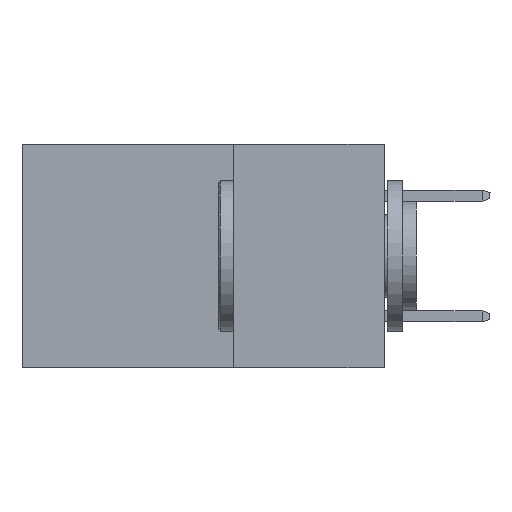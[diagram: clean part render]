
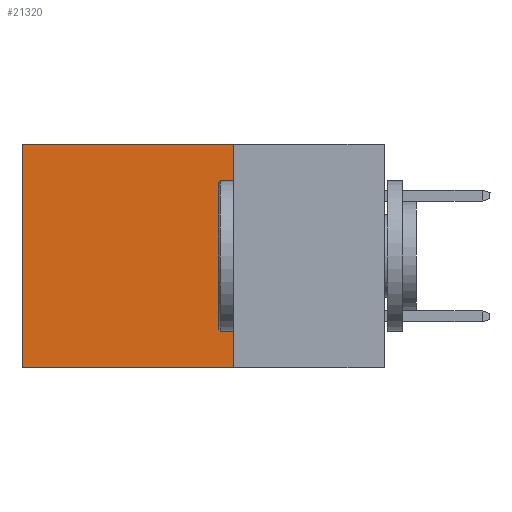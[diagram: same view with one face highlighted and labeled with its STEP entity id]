
A CAD part, left-side view. The second image highlights one B-rep face of the part: STEP entity #21320.
In plain terms, the highlighted planar face has unit normal (-1, 0, 0).
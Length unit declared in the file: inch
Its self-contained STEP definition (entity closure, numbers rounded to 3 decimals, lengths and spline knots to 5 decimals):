
#427 = DIRECTION ( 'NONE',  ( 0., 0., -1. ) ) ;
#966 = LINE ( 'NONE', #11184, #6927 ) ;
#1283 = ORIENTED_EDGE ( 'NONE', *, *, #21250, .F. ) ;
#1818 = DIRECTION ( 'NONE',  ( 1., 0., 0. ) ) ;
#2994 = LINE ( 'NONE', #25453, #27634 ) ;
#3259 = CARTESIAN_POINT ( 'NONE',  ( 0.298, 0.25, -0.37 ) ) ;
#6927 = VECTOR ( 'NONE', #10990, 39.37008 ) ;
#7631 = EDGE_CURVE ( 'NONE', #20984, #27270, #966, .T. ) ;
#8198 = ORIENTED_EDGE ( 'NONE', *, *, #16714, .F. ) ;
#10990 = DIRECTION ( 'NONE',  ( 0., 0., -1. ) ) ;
#11184 = CARTESIAN_POINT ( 'NONE',  ( 0.298, 0.6, 0. ) ) ;
#11274 = FACE_OUTER_BOUND ( 'NONE', #28308, .T. ) ;
#11840 = CARTESIAN_POINT ( 'NONE',  ( 0.298, 0.25, 0. ) ) ;
#12133 = CARTESIAN_POINT ( 'NONE',  ( 0.298, 0.25, 0. ) ) ;
#13367 = DIRECTION ( 'NONE',  ( 0., 1., 0. ) ) ;
#13793 = EDGE_CURVE ( 'NONE', #16463, #20984, #2994, .T. ) ;
#14115 = DIRECTION ( 'NONE',  ( 0., 1., 0. ) ) ;
#14314 = PLANE ( 'NONE',  #24502 ) ;
#16141 = VERTEX_POINT ( 'NONE', #3259 ) ;
#16449 = CARTESIAN_POINT ( 'NONE',  ( 0.298, 0.25, -0.37 ) ) ;
#16463 = VERTEX_POINT ( 'NONE', #12133 ) ;
#16714 = EDGE_CURVE ( 'NONE', #16463, #16141, #24123, .T. ) ;
#17716 = VECTOR ( 'NONE', #427, 39.37008 ) ;
#17915 = CARTESIAN_POINT ( 'NONE',  ( 0.298, 0.25, 0. ) ) ;
#19197 = DIRECTION ( 'NONE',  ( 0., 0., -1. ) ) ;
#19315 = LINE ( 'NONE', #16449, #25004 ) ;
#20984 = VERTEX_POINT ( 'NONE', #25153 ) ;
#21250 = EDGE_CURVE ( 'NONE', #16141, #27270, #19315, .T. ) ;
#21320 = ADVANCED_FACE ( 'NONE', ( #11274 ), #14314, .F. ) ;
#23190 = CARTESIAN_POINT ( 'NONE',  ( 0.298, 0.6, -0.37 ) ) ;
#24123 = LINE ( 'NONE', #17915, #17716 ) ;
#24502 = AXIS2_PLACEMENT_3D ( 'NONE', #11840, #1818, #19197 ) ;
#25004 = VECTOR ( 'NONE', #14115, 39.37008 ) ;
#25153 = CARTESIAN_POINT ( 'NONE',  ( 0.298, 0.6, 0. ) ) ;
#25453 = CARTESIAN_POINT ( 'NONE',  ( 0.298, 0.25, 0. ) ) ;
#26979 = ORIENTED_EDGE ( 'NONE', *, *, #7631, .T. ) ;
#27270 = VERTEX_POINT ( 'NONE', #23190 ) ;
#27634 = VECTOR ( 'NONE', #13367, 39.37008 ) ;
#28308 = EDGE_LOOP ( 'NONE', ( #26979, #1283, #8198, #29389 ) ) ;
#29389 = ORIENTED_EDGE ( 'NONE', *, *, #13793, .T. ) ;
